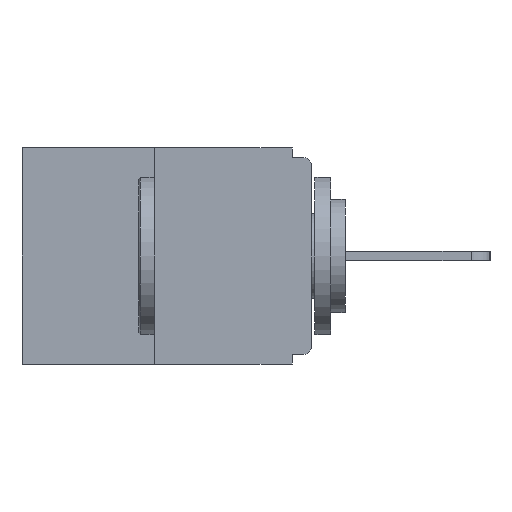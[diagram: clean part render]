
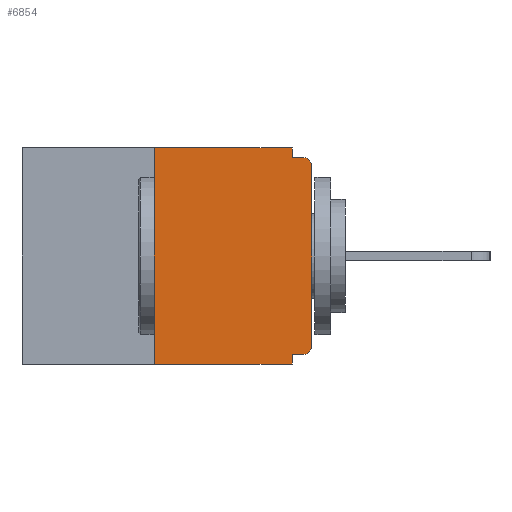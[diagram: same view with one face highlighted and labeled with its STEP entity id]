
A CAD part, left-side view. The second image highlights one B-rep face of the part: STEP entity #6854.
In plain terms, the highlighted planar face has unit normal (-1, 0, 0).
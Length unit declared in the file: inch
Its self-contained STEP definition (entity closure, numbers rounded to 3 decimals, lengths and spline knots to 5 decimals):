
#39 = DIRECTION ( 'NONE',  ( 0., 1., 0. ) ) ;
#84 = VECTOR ( 'NONE', #14342, 39.37008 ) ;
#105 = VERTEX_POINT ( 'NONE', #16360 ) ;
#156 = FACE_OUTER_BOUND ( 'NONE', #319, .T. ) ;
#319 = EDGE_LOOP ( 'NONE', ( #7654, #17101, #8480, #8430, #19002, #4447, #15770, #6944, #10245, #6082 ) ) ;
#339 = DIRECTION ( 'NONE',  ( 0., 0., 1. ) ) ;
#433 = VECTOR ( 'NONE', #3934, 39.37008 ) ;
#726 = CARTESIAN_POINT ( 'NONE',  ( 0., 0., 0. ) ) ;
#832 = EDGE_CURVE ( 'NONE', #16640, #17389, #18404, .T. ) ;
#933 = CARTESIAN_POINT ( 'NONE',  ( 0., 0.46, -0.343 ) ) ;
#1406 = VECTOR ( 'NONE', #339, 39.37008 ) ;
#1425 = CARTESIAN_POINT ( 'NONE',  ( 0., 0., -0.328 ) ) ;
#1919 = VECTOR ( 'NONE', #39, 39.37008 ) ;
#2037 = CIRCLE ( 'NONE', #4071, 0.015 ) ;
#2155 = LINE ( 'NONE', #13433, #8703 ) ;
#2316 = CARTESIAN_POINT ( 'NONE',  ( 0., 0.46, 0. ) ) ;
#2409 = CARTESIAN_POINT ( 'NONE',  ( 0., 0.031, -0.343 ) ) ;
#2935 = DIRECTION ( 'NONE',  ( 1., 0., 0. ) ) ;
#3050 = EDGE_CURVE ( 'NONE', #6618, #4142, #2155, .T. ) ;
#3483 = CARTESIAN_POINT ( 'NONE',  ( 0., 0.031, -0.343 ) ) ;
#3750 = VECTOR ( 'NONE', #5777, 39.37008 ) ;
#3814 = DIRECTION ( 'NONE',  ( 0., -1., 0. ) ) ;
#3889 = CARTESIAN_POINT ( 'NONE',  ( 0., 0.015, -0.015 ) ) ;
#3934 = DIRECTION ( 'NONE',  ( 0., 0., -1. ) ) ;
#4071 = AXIS2_PLACEMENT_3D ( 'NONE', #13573, #11669, #7118 ) ;
#4142 = VERTEX_POINT ( 'NONE', #3889 ) ;
#4447 = ORIENTED_EDGE ( 'NONE', *, *, #7797, .T. ) ;
#4545 = EDGE_CURVE ( 'NONE', #10682, #6618, #15305, .T. ) ;
#4579 = EDGE_CURVE ( 'NONE', #10344, #105, #13195, .T. ) ;
#5362 = VERTEX_POINT ( 'NONE', #6459 ) ;
#5432 = VECTOR ( 'NONE', #3814, 39.37008 ) ;
#5777 = DIRECTION ( 'NONE',  ( 0., 0., 1. ) ) ;
#6082 = ORIENTED_EDGE ( 'NONE', *, *, #4545, .F. ) ;
#6338 = LINE ( 'NONE', #7761, #1406 ) ;
#6459 = CARTESIAN_POINT ( 'NONE',  ( 0., 0.015, -0.328 ) ) ;
#6618 = VERTEX_POINT ( 'NONE', #17234 ) ;
#6738 = DIRECTION ( 'NONE',  ( 0., 0., -1. ) ) ;
#6854 = ADVANCED_FACE ( 'NONE', ( #156 ), #10208, .F. ) ;
#6944 = ORIENTED_EDGE ( 'NONE', *, *, #13905, .T. ) ;
#7118 = DIRECTION ( 'NONE',  ( 0., 0., -1. ) ) ;
#7455 = DIRECTION ( 'NONE',  ( 0., 0., -1. ) ) ;
#7654 = ORIENTED_EDGE ( 'NONE', *, *, #15523, .F. ) ;
#7761 = CARTESIAN_POINT ( 'NONE',  ( 0., 0.25, 0. ) ) ;
#7797 = EDGE_CURVE ( 'NONE', #5362, #10344, #15420, .T. ) ;
#8430 = ORIENTED_EDGE ( 'NONE', *, *, #12261, .F. ) ;
#8480 = ORIENTED_EDGE ( 'NONE', *, *, #832, .T. ) ;
#8703 = VECTOR ( 'NONE', #9002, 39.37008 ) ;
#9002 = DIRECTION ( 'NONE',  ( 0., -1., 0. ) ) ;
#9350 = CARTESIAN_POINT ( 'NONE',  ( 0., 0.031, -0.328 ) ) ;
#9378 = LINE ( 'NONE', #2409, #433 ) ;
#9979 = EDGE_CURVE ( 'NONE', #5362, #11415, #10380, .T. ) ;
#10208 = PLANE ( 'NONE',  #15577 ) ;
#10245 = ORIENTED_EDGE ( 'NONE', *, *, #3050, .F. ) ;
#10344 = VERTEX_POINT ( 'NONE', #13911 ) ;
#10380 = LINE ( 'NONE', #1425, #1919 ) ;
#10682 = VERTEX_POINT ( 'NONE', #12578 ) ;
#11042 = DIRECTION ( 'NONE',  ( -1., 0., 0. ) ) ;
#11415 = VERTEX_POINT ( 'NONE', #9350 ) ;
#11629 = EDGE_CURVE ( 'NONE', #16640, #13605, #6338, .T. ) ;
#11669 = DIRECTION ( 'NONE',  ( -1., 0., 0. ) ) ;
#12261 = EDGE_CURVE ( 'NONE', #11415, #17389, #9378, .T. ) ;
#12422 = AXIS2_PLACEMENT_3D ( 'NONE', #15734, #11042, #15668 ) ;
#12578 = CARTESIAN_POINT ( 'NONE',  ( 0., 0.031, 0. ) ) ;
#13195 = LINE ( 'NONE', #726, #3750 ) ;
#13433 = CARTESIAN_POINT ( 'NONE',  ( 0., 0., -0.015 ) ) ;
#13573 = CARTESIAN_POINT ( 'NONE',  ( 0., 0.015, -0.03 ) ) ;
#13605 = VERTEX_POINT ( 'NONE', #18962 ) ;
#13905 = EDGE_CURVE ( 'NONE', #105, #4142, #2037, .T. ) ;
#13911 = CARTESIAN_POINT ( 'NONE',  ( 0., 0., -0.313 ) ) ;
#14342 = DIRECTION ( 'NONE',  ( 0., -1., 0. ) ) ;
#14427 = LINE ( 'NONE', #2316, #84 ) ;
#14767 = CARTESIAN_POINT ( 'NONE',  ( 0., 0.46, 0. ) ) ;
#15067 = CARTESIAN_POINT ( 'NONE',  ( 0., 0.25, -0.343 ) ) ;
#15305 = LINE ( 'NONE', #17376, #16761 ) ;
#15420 = CIRCLE ( 'NONE', #12422, 0.015 ) ;
#15523 = EDGE_CURVE ( 'NONE', #13605, #10682, #14427, .T. ) ;
#15577 = AXIS2_PLACEMENT_3D ( 'NONE', #14767, #2935, #7455 ) ;
#15668 = DIRECTION ( 'NONE',  ( 0., 0., -1. ) ) ;
#15734 = CARTESIAN_POINT ( 'NONE',  ( 0., 0.015, -0.313 ) ) ;
#15770 = ORIENTED_EDGE ( 'NONE', *, *, #4579, .T. ) ;
#16360 = CARTESIAN_POINT ( 'NONE',  ( 0., 0., -0.03 ) ) ;
#16640 = VERTEX_POINT ( 'NONE', #15067 ) ;
#16761 = VECTOR ( 'NONE', #6738, 39.37008 ) ;
#17101 = ORIENTED_EDGE ( 'NONE', *, *, #11629, .F. ) ;
#17234 = CARTESIAN_POINT ( 'NONE',  ( 0., 0.031, -0.015 ) ) ;
#17376 = CARTESIAN_POINT ( 'NONE',  ( 0., 0.031, 0. ) ) ;
#17389 = VERTEX_POINT ( 'NONE', #3483 ) ;
#18404 = LINE ( 'NONE', #933, #5432 ) ;
#18962 = CARTESIAN_POINT ( 'NONE',  ( 0., 0.25, 0. ) ) ;
#19002 = ORIENTED_EDGE ( 'NONE', *, *, #9979, .F. ) ;
